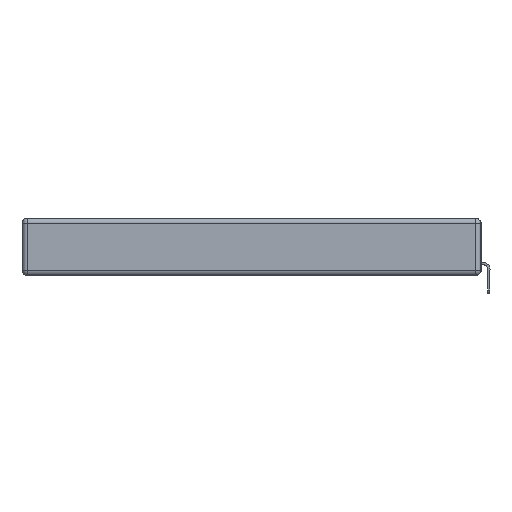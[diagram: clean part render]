
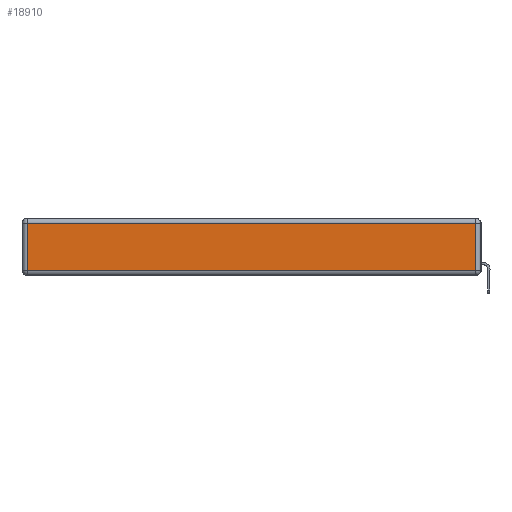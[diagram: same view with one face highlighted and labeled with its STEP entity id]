
A CAD part, left-side view. The second image highlights one B-rep face of the part: STEP entity #18910.
In plain terms, the highlighted planar face has unit normal (-1, 0, 0).
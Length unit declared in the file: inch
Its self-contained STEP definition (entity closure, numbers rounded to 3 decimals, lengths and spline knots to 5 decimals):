
#240 = DIRECTION ( 'NONE',  ( -1., 0., 0. ) ) ;
#840 = EDGE_CURVE ( 'NONE', #7999, #19040, #11758, .T. ) ;
#983 = EDGE_LOOP ( 'NONE', ( #17293, #2813, #9081, #19788 ) ) ;
#1026 = DIRECTION ( 'NONE',  ( 0., 0., -1. ) ) ;
#2009 = VECTOR ( 'NONE', #1026, 39.37008 ) ;
#2179 = VECTOR ( 'NONE', #16748, 39.37008 ) ;
#2683 = CARTESIAN_POINT ( 'NONE',  ( 0., 0.03, -0.343 ) ) ;
#2811 = LINE ( 'NONE', #2683, #15516 ) ;
#2813 = ORIENTED_EDGE ( 'NONE', *, *, #15404, .T. ) ;
#3007 = CARTESIAN_POINT ( 'NONE',  ( 0., 0.03, -0.313 ) ) ;
#4310 = FACE_OUTER_BOUND ( 'NONE', #983, .T. ) ;
#4322 = DIRECTION ( 'NONE',  ( 0., 0., 1. ) ) ;
#5456 = VECTOR ( 'NONE', #11521, 39.37008 ) ;
#6067 = LINE ( 'NONE', #16402, #2009 ) ;
#7216 = CARTESIAN_POINT ( 'NONE',  ( 0., 2.72, -0.313 ) ) ;
#7463 = CARTESIAN_POINT ( 'NONE',  ( 0., 0., -0.313 ) ) ;
#7999 = VERTEX_POINT ( 'NONE', #7216 ) ;
#8009 = EDGE_CURVE ( 'NONE', #14966, #7999, #6067, .T. ) ;
#9081 = ORIENTED_EDGE ( 'NONE', *, *, #12505, .T. ) ;
#9377 = PLANE ( 'NONE',  #19607 ) ;
#9442 = CARTESIAN_POINT ( 'NONE',  ( 0., 0., -0.343 ) ) ;
#10950 = LINE ( 'NONE', #15965, #5456 ) ;
#11502 = CARTESIAN_POINT ( 'NONE',  ( 0., 0.03, -0.03 ) ) ;
#11521 = DIRECTION ( 'NONE',  ( 0., 1., 0. ) ) ;
#11758 = LINE ( 'NONE', #7463, #2179 ) ;
#12505 = EDGE_CURVE ( 'NONE', #19265, #14966, #10950, .T. ) ;
#13814 = CARTESIAN_POINT ( 'NONE',  ( 0., 2.72, -0.03 ) ) ;
#14966 = VERTEX_POINT ( 'NONE', #13814 ) ;
#15404 = EDGE_CURVE ( 'NONE', #19040, #19265, #2811, .T. ) ;
#15516 = VECTOR ( 'NONE', #4322, 39.37008 ) ;
#15965 = CARTESIAN_POINT ( 'NONE',  ( 0., 2.75, -0.03 ) ) ;
#16402 = CARTESIAN_POINT ( 'NONE',  ( 0., 2.72, -0.343 ) ) ;
#16748 = DIRECTION ( 'NONE',  ( 0., -1., 0. ) ) ;
#17155 = DIRECTION ( 'NONE',  ( 0., 0., 1. ) ) ;
#17293 = ORIENTED_EDGE ( 'NONE', *, *, #840, .T. ) ;
#18910 = ADVANCED_FACE ( 'NONE', ( #4310 ), #9377, .T. ) ;
#19040 = VERTEX_POINT ( 'NONE', #3007 ) ;
#19265 = VERTEX_POINT ( 'NONE', #11502 ) ;
#19607 = AXIS2_PLACEMENT_3D ( 'NONE', #9442, #240, #17155 ) ;
#19788 = ORIENTED_EDGE ( 'NONE', *, *, #8009, .T. ) ;
